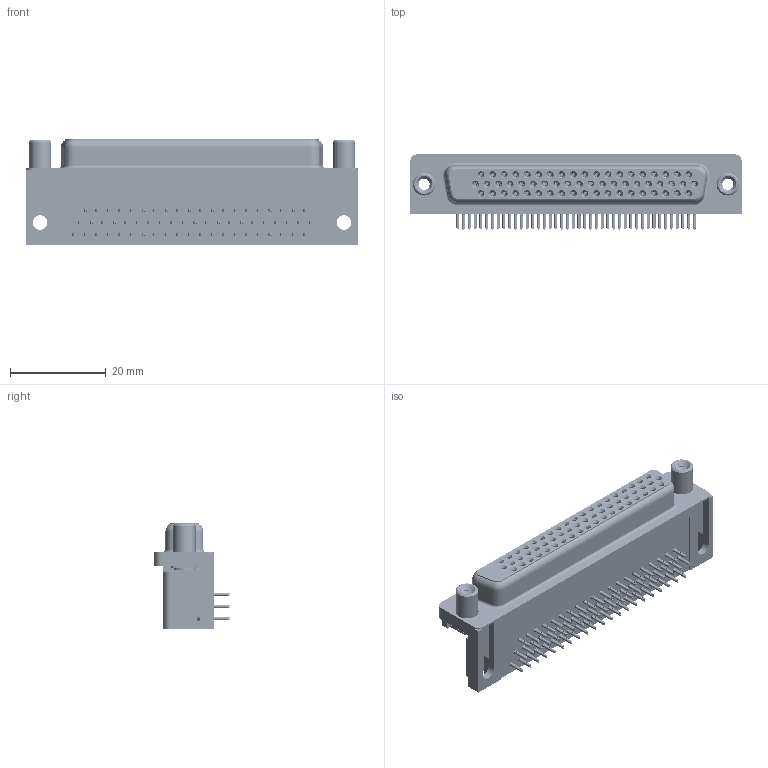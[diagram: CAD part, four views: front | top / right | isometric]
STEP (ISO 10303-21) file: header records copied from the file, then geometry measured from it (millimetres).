
FILE_DESCRIPTION (( 'STEP AP203' ), '1' );
FILE_NAME ('634-062-263-010.STEP', '2018-08-21T18:54:05', ( '' ), ( '' ), 'SwSTEP 2.0', 'SolidWorks 2016', '' );
FILE_SCHEMA (( 'CONFIG_CONTROL_DESIGN' ));
Length unit declared in the file: millimetre
Products named in the file (8): 634 Housing_62 Socket; 634 Shell_62 Socket; Contact Bottom; Contact Middle; Contact Top; Thru Hole Board Mount; Round Threaded Standoff; 634-062-263-010
Assembly tree (68 placements, depth 2):
  634-062-263-010
    634 Housing_62 Socket
    634 Shell_62 Socket
    Contact Bottom  x20
    Contact Middle  x21
    Contact Top  x21
    Thru Hole Board Mount  x2
    Round Threaded Standoff  x2
Bounding box: 69.4 x 15.73 x 22.1 mm (x, y, z)
Volume: 13031.9 mm3; surface area: 17938.9 mm2
Topology: 72 solids, 72 shells, 9089 faces, 23900 edges, 14998 vertices
Faces by surface type: plane 4081, bspline 2168, cylinder 2062, cone 756, torus 22
Entity records: 52912 total; most frequent: CARTESIAN_POINT 15036, ORIENTED_EDGE 7402, DIRECTION 6931, EDGE_CURVE 3701, VECTOR 2577, LINE 2577, VERTEX_POINT 2372, AXIS2_PLACEMENT_3D 2177
